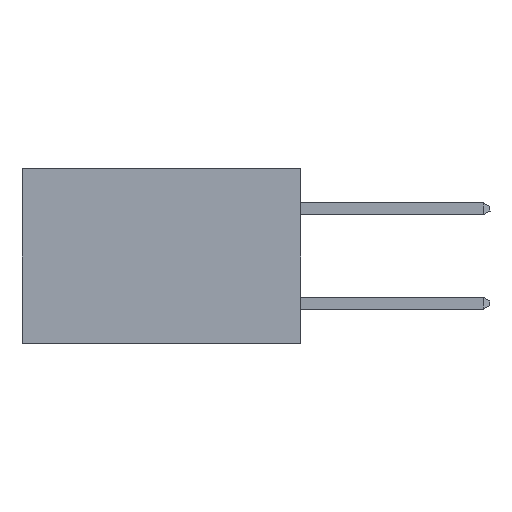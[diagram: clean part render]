
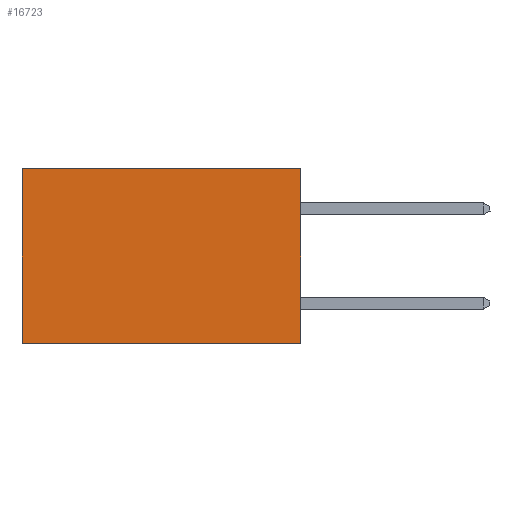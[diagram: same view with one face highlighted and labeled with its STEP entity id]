
A CAD part, left-side view. The second image highlights one B-rep face of the part: STEP entity #16723.
In plain terms, the highlighted planar face has unit normal (-1, 0, 0).
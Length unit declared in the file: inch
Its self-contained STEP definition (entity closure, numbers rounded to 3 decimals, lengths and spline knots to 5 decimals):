
#1597 = DIRECTION ( 'NONE',  ( 0., 1., 0. ) ) ;
#2258 = EDGE_CURVE ( 'NONE', #24820, #7267, #6101, .T. ) ;
#2534 = EDGE_CURVE ( 'NONE', #4970, #7267, #14806, .T. ) ;
#2616 = AXIS2_PLACEMENT_3D ( 'NONE', #10593, #18812, #6510 ) ;
#3333 = CARTESIAN_POINT ( 'NONE',  ( 0.277, 0., 0. ) ) ;
#4970 = VERTEX_POINT ( 'NONE', #20594 ) ;
#5463 = VECTOR ( 'NONE', #1597, 39.37008 ) ;
#5471 = EDGE_LOOP ( 'NONE', ( #24832, #14973, #7521, #22982 ) ) ;
#6101 = LINE ( 'NONE', #14771, #5463 ) ;
#6341 = DIRECTION ( 'NONE',  ( 0., 0., -1. ) ) ;
#6510 = DIRECTION ( 'NONE',  ( 0., 0., -1. ) ) ;
#7267 = VERTEX_POINT ( 'NONE', #9079 ) ;
#7521 = ORIENTED_EDGE ( 'NONE', *, *, #10614, .F. ) ;
#8158 = CARTESIAN_POINT ( 'NONE',  ( 0.277, 0.59, -0.37 ) ) ;
#9079 = CARTESIAN_POINT ( 'NONE',  ( 0.277, 0.59, -0.37 ) ) ;
#10593 = CARTESIAN_POINT ( 'NONE',  ( 0.277, 0., -0.37 ) ) ;
#10614 = EDGE_CURVE ( 'NONE', #19054, #24820, #16705, .T. ) ;
#10844 = CARTESIAN_POINT ( 'NONE',  ( 0.277, 0., 0. ) ) ;
#11255 = VECTOR ( 'NONE', #6341, 39.37008 ) ;
#11935 = EDGE_CURVE ( 'NONE', #19054, #4970, #24001, .T. ) ;
#12559 = CARTESIAN_POINT ( 'NONE',  ( 0.277, 0., -0.37 ) ) ;
#12881 = DIRECTION ( 'NONE',  ( 0., 1., 0. ) ) ;
#14727 = PLANE ( 'NONE',  #2616 ) ;
#14771 = CARTESIAN_POINT ( 'NONE',  ( 0.277, 0., -0.37 ) ) ;
#14806 = LINE ( 'NONE', #8158, #20225 ) ;
#14973 = ORIENTED_EDGE ( 'NONE', *, *, #2258, .F. ) ;
#16705 = LINE ( 'NONE', #12559, #11255 ) ;
#16723 = ADVANCED_FACE ( 'NONE', ( #19105 ), #14727, .F. ) ;
#18812 = DIRECTION ( 'NONE',  ( 1., 0., 0. ) ) ;
#19054 = VERTEX_POINT ( 'NONE', #3333 ) ;
#19105 = FACE_OUTER_BOUND ( 'NONE', #5471, .T. ) ;
#19474 = CARTESIAN_POINT ( 'NONE',  ( 0.277, 0., -0.37 ) ) ;
#20225 = VECTOR ( 'NONE', #22917, 39.37008 ) ;
#20594 = CARTESIAN_POINT ( 'NONE',  ( 0.277, 0.59, 0. ) ) ;
#22101 = VECTOR ( 'NONE', #12881, 39.37008 ) ;
#22917 = DIRECTION ( 'NONE',  ( 0., 0., -1. ) ) ;
#22982 = ORIENTED_EDGE ( 'NONE', *, *, #11935, .T. ) ;
#24001 = LINE ( 'NONE', #10844, #22101 ) ;
#24820 = VERTEX_POINT ( 'NONE', #19474 ) ;
#24832 = ORIENTED_EDGE ( 'NONE', *, *, #2534, .T. ) ;
